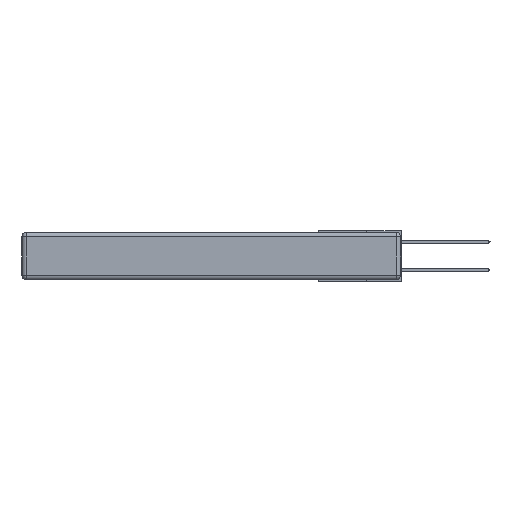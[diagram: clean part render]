
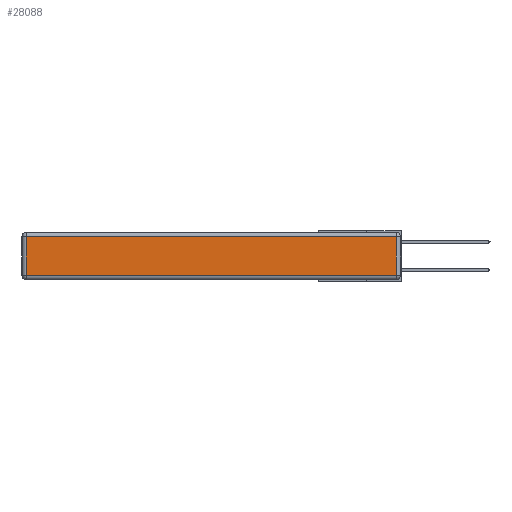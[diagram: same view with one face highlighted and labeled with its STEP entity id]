
A CAD part, left-side view. The second image highlights one B-rep face of the part: STEP entity #28088.
In plain terms, the highlighted planar face has unit normal (-1, 0, 0).
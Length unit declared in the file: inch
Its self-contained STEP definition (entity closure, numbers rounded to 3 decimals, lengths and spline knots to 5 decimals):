
#164 = DIRECTION ( 'NONE',  ( -1., 0., 0. ) ) ;
#2441 = DIRECTION ( 'NONE',  ( 0., 0., 1. ) ) ;
#2706 = DIRECTION ( 'NONE',  ( 0., 1., 0. ) ) ;
#2826 = CARTESIAN_POINT ( 'NONE',  ( 0., 2.72, -0.03 ) ) ;
#6026 = CARTESIAN_POINT ( 'NONE',  ( 0., 0., -0.313 ) ) ;
#6162 = FACE_OUTER_BOUND ( 'NONE', #10632, .T. ) ;
#6212 = ORIENTED_EDGE ( 'NONE', *, *, #16466, .T. ) ;
#6243 = EDGE_CURVE ( 'NONE', #29345, #7631, #9730, .T. ) ;
#6411 = LINE ( 'NONE', #28063, #7829 ) ;
#7631 = VERTEX_POINT ( 'NONE', #15943 ) ;
#7829 = VECTOR ( 'NONE', #2706, 39.37008 ) ;
#9730 = LINE ( 'NONE', #12826, #20805 ) ;
#10334 = ORIENTED_EDGE ( 'NONE', *, *, #6243, .T. ) ;
#10632 = EDGE_LOOP ( 'NONE', ( #6212, #10334, #17029, #20834 ) ) ;
#12714 = EDGE_CURVE ( 'NONE', #7631, #17809, #6411, .T. ) ;
#12826 = CARTESIAN_POINT ( 'NONE',  ( 0., 0.03, -0.343 ) ) ;
#12920 = DIRECTION ( 'NONE',  ( 0., -1., 0. ) ) ;
#13776 = CARTESIAN_POINT ( 'NONE',  ( 0., 2.72, -0.313 ) ) ;
#15943 = CARTESIAN_POINT ( 'NONE',  ( 0., 0.03, -0.03 ) ) ;
#15967 = CARTESIAN_POINT ( 'NONE',  ( 0., 0.03, -0.313 ) ) ;
#16000 = EDGE_CURVE ( 'NONE', #17809, #21362, #25547, .T. ) ;
#16466 = EDGE_CURVE ( 'NONE', #21362, #29345, #28760, .T. ) ;
#17029 = ORIENTED_EDGE ( 'NONE', *, *, #12714, .T. ) ;
#17809 = VERTEX_POINT ( 'NONE', #2826 ) ;
#18318 = CARTESIAN_POINT ( 'NONE',  ( 0., 0., -0.343 ) ) ;
#19489 = VECTOR ( 'NONE', #12920, 39.37008 ) ;
#20805 = VECTOR ( 'NONE', #26404, 39.37008 ) ;
#20834 = ORIENTED_EDGE ( 'NONE', *, *, #16000, .T. ) ;
#21362 = VERTEX_POINT ( 'NONE', #13776 ) ;
#21497 = AXIS2_PLACEMENT_3D ( 'NONE', #18318, #164, #2441 ) ;
#21623 = VECTOR ( 'NONE', #29320, 39.37008 ) ;
#25547 = LINE ( 'NONE', #28933, #21623 ) ;
#26404 = DIRECTION ( 'NONE',  ( 0., 0., 1. ) ) ;
#27603 = PLANE ( 'NONE',  #21497 ) ;
#28063 = CARTESIAN_POINT ( 'NONE',  ( 0., 2.75, -0.03 ) ) ;
#28088 = ADVANCED_FACE ( 'NONE', ( #6162 ), #27603, .T. ) ;
#28760 = LINE ( 'NONE', #6026, #19489 ) ;
#28933 = CARTESIAN_POINT ( 'NONE',  ( 0., 2.72, -0.343 ) ) ;
#29320 = DIRECTION ( 'NONE',  ( 0., 0., -1. ) ) ;
#29345 = VERTEX_POINT ( 'NONE', #15967 ) ;
